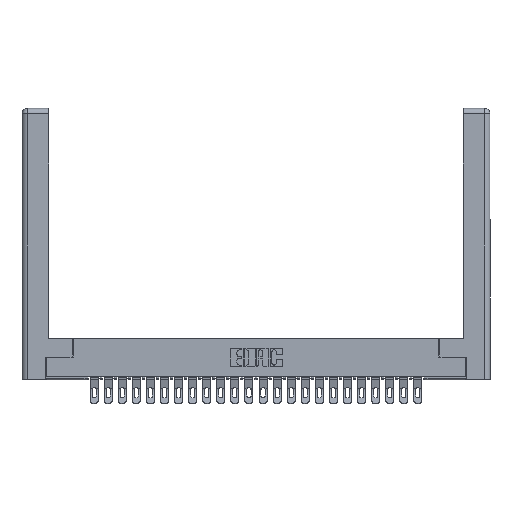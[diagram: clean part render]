
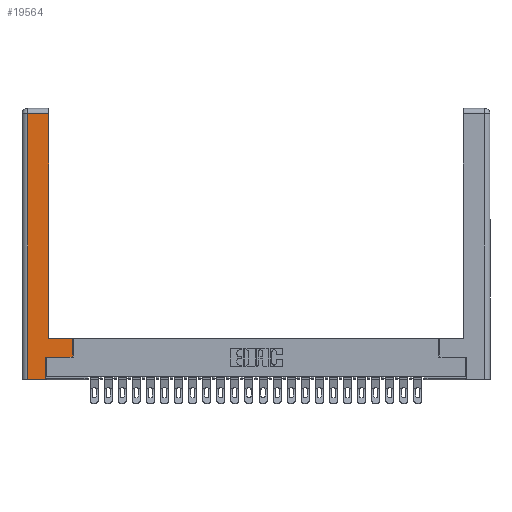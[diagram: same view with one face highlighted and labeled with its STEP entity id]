
A CAD part, top view. The second image highlights one B-rep face of the part: STEP entity #19564.
In plain terms, the highlighted planar face has unit normal (0, 0, 1).
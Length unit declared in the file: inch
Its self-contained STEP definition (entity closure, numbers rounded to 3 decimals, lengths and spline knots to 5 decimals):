
#861 = ORIENTED_EDGE ( 'NONE', *, *, #26148, .T. ) ;
#880 = VECTOR ( 'NONE', #4112, 39.37008 ) ;
#1448 = CARTESIAN_POINT ( 'NONE',  ( 0.0615, 2.94, 0. ) ) ;
#2400 = VERTEX_POINT ( 'NONE', #21656 ) ;
#2410 = EDGE_CURVE ( 'NONE', #10834, #17080, #17279, .T. ) ;
#2751 = CARTESIAN_POINT ( 'NONE',  ( 0.265, 0., 0. ) ) ;
#3232 = VECTOR ( 'NONE', #12876, 39.37008 ) ;
#3732 = CARTESIAN_POINT ( 'NONE',  ( 0.295, 2.94, 0. ) ) ;
#4056 = FACE_OUTER_BOUND ( 'NONE', #11852, .T. ) ;
#4112 = DIRECTION ( 'NONE',  ( 1., 0., 0. ) ) ;
#4562 = VERTEX_POINT ( 'NONE', #2751 ) ;
#4600 = LINE ( 'NONE', #24981, #16730 ) ;
#5148 = VECTOR ( 'NONE', #18764, 39.37008 ) ;
#5861 = EDGE_CURVE ( 'NONE', #17080, #4562, #28940, .T. ) ;
#7138 = LINE ( 'NONE', #12863, #24153 ) ;
#7254 = VECTOR ( 'NONE', #28510, 39.37008 ) ;
#8270 = ORIENTED_EDGE ( 'NONE', *, *, #5861, .T. ) ;
#8457 = DIRECTION ( 'NONE',  ( 0., 1., 0. ) ) ;
#8555 = EDGE_CURVE ( 'NONE', #2400, #28319, #7138, .T. ) ;
#9197 = VECTOR ( 'NONE', #13534, 39.37008 ) ;
#10422 = CARTESIAN_POINT ( 'NONE',  ( 0.0615, 2.94, 0. ) ) ;
#10479 = DIRECTION ( 'NONE',  ( -1., 0., 0. ) ) ;
#10834 = VERTEX_POINT ( 'NONE', #1448 ) ;
#11480 = LINE ( 'NONE', #28650, #9197 ) ;
#11852 = EDGE_LOOP ( 'NONE', ( #861, #18443, #17563, #8270, #12456, #23455, #16841, #25793 ) ) ;
#12456 = ORIENTED_EDGE ( 'NONE', *, *, #21502, .T. ) ;
#12863 = CARTESIAN_POINT ( 'NONE',  ( 0.565, 0.245, 0. ) ) ;
#12876 = DIRECTION ( 'NONE',  ( -1., 0., 0. ) ) ;
#13534 = DIRECTION ( 'NONE',  ( 0., 1., 0. ) ) ;
#13683 = LINE ( 'NONE', #23395, #7254 ) ;
#14321 = DIRECTION ( 'NONE',  ( 0., 0., -1. ) ) ;
#14726 = CARTESIAN_POINT ( 'NONE',  ( 0.0615, 0., 0. ) ) ;
#15812 = AXIS2_PLACEMENT_3D ( 'NONE', #28397, #14321, #27371 ) ;
#16730 = VECTOR ( 'NONE', #10479, 39.37008 ) ;
#16841 = ORIENTED_EDGE ( 'NONE', *, *, #24864, .T. ) ;
#17080 = VERTEX_POINT ( 'NONE', #14726 ) ;
#17279 = LINE ( 'NONE', #21025, #5148 ) ;
#17563 = ORIENTED_EDGE ( 'NONE', *, *, #2410, .T. ) ;
#17740 = CARTESIAN_POINT ( 'NONE',  ( 0.565, 0.45, 0. ) ) ;
#18443 = ORIENTED_EDGE ( 'NONE', *, *, #28432, .T. ) ;
#18764 = DIRECTION ( 'NONE',  ( 0., -1., 0. ) ) ;
#19564 = ADVANCED_FACE ( 'NONE', ( #4056 ), #30733, .F. ) ;
#21025 = CARTESIAN_POINT ( 'NONE',  ( 0.0615, 0., 0. ) ) ;
#21502 = EDGE_CURVE ( 'NONE', #4562, #2400, #11480, .T. ) ;
#21656 = CARTESIAN_POINT ( 'NONE',  ( 0.265, 0.245, 0. ) ) ;
#21997 = VERTEX_POINT ( 'NONE', #28656 ) ;
#22660 = LINE ( 'NONE', #30120, #31059 ) ;
#23395 = CARTESIAN_POINT ( 'NONE',  ( 0.565, 0.45, 0. ) ) ;
#23455 = ORIENTED_EDGE ( 'NONE', *, *, #8555, .T. ) ;
#24153 = VECTOR ( 'NONE', #25022, 39.37008 ) ;
#24830 = EDGE_CURVE ( 'NONE', #25825, #21997, #4600, .T. ) ;
#24864 = EDGE_CURVE ( 'NONE', #28319, #25825, #13683, .T. ) ;
#24981 = CARTESIAN_POINT ( 'NONE',  ( 0.295, 0.45, 0. ) ) ;
#25022 = DIRECTION ( 'NONE',  ( 1., 0., 0. ) ) ;
#25793 = ORIENTED_EDGE ( 'NONE', *, *, #24830, .T. ) ;
#25825 = VERTEX_POINT ( 'NONE', #17740 ) ;
#26031 = CARTESIAN_POINT ( 'NONE',  ( 0.265, 0., 0. ) ) ;
#26148 = EDGE_CURVE ( 'NONE', #21997, #29492, #22660, .T. ) ;
#27371 = DIRECTION ( 'NONE',  ( -1., 0., 0. ) ) ;
#28319 = VERTEX_POINT ( 'NONE', #30997 ) ;
#28397 = CARTESIAN_POINT ( 'NONE',  ( 0., 0., 0. ) ) ;
#28432 = EDGE_CURVE ( 'NONE', #29492, #10834, #30168, .T. ) ;
#28510 = DIRECTION ( 'NONE',  ( 0., 1., 0. ) ) ;
#28650 = CARTESIAN_POINT ( 'NONE',  ( 0.265, 0.245, 0. ) ) ;
#28656 = CARTESIAN_POINT ( 'NONE',  ( 0.295, 0.45, 0. ) ) ;
#28940 = LINE ( 'NONE', #26031, #880 ) ;
#29492 = VERTEX_POINT ( 'NONE', #3732 ) ;
#30120 = CARTESIAN_POINT ( 'NONE',  ( 0.295, 3., 0. ) ) ;
#30168 = LINE ( 'NONE', #10422, #3232 ) ;
#30733 = PLANE ( 'NONE',  #15812 ) ;
#30997 = CARTESIAN_POINT ( 'NONE',  ( 0.565, 0.245, 0. ) ) ;
#31059 = VECTOR ( 'NONE', #8457, 39.37008 ) ;
